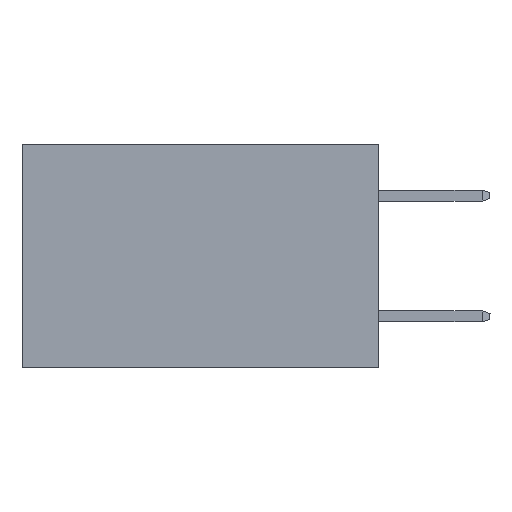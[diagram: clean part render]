
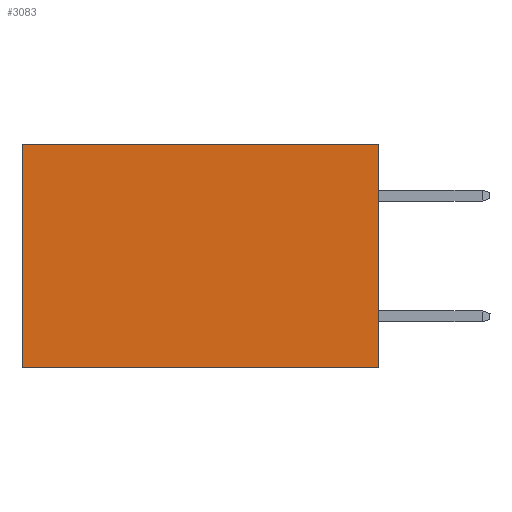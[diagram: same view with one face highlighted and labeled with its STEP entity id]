
A CAD part, left-side view. The second image highlights one B-rep face of the part: STEP entity #3083.
In plain terms, the highlighted planar face has unit normal (-1, 0, 0).
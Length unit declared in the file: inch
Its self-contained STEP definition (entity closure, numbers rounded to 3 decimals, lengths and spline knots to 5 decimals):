
#747 = DIRECTION ( 'NONE',  ( 0., 0., -1. ) ) ;
#791 = LINE ( 'NONE', #6484, #8474 ) ;
#910 = CARTESIAN_POINT ( 'NONE',  ( 0.277, 0.59, -0.37 ) ) ;
#1639 = CARTESIAN_POINT ( 'NONE',  ( 0.277, 0., -0.37 ) ) ;
#1869 = EDGE_CURVE ( 'NONE', #4061, #5436, #791, .T. ) ;
#1875 = VECTOR ( 'NONE', #5075, 39.37008 ) ;
#2324 = LINE ( 'NONE', #5632, #4254 ) ;
#2449 = EDGE_LOOP ( 'NONE', ( #4635, #6567, #8418, #2709 ) ) ;
#2709 = ORIENTED_EDGE ( 'NONE', *, *, #1869, .T. ) ;
#2907 = VECTOR ( 'NONE', #747, 39.37008 ) ;
#3083 = ADVANCED_FACE ( 'NONE', ( #7697 ), #7698, .F. ) ;
#3632 = AXIS2_PLACEMENT_3D ( 'NONE', #7762, #5878, #5810 ) ;
#3664 = EDGE_CURVE ( 'NONE', #4647, #9461, #2324, .T. ) ;
#3695 = EDGE_CURVE ( 'NONE', #4061, #4647, #6456, .T. ) ;
#4061 = VERTEX_POINT ( 'NONE', #4425 ) ;
#4254 = VECTOR ( 'NONE', #5204, 39.37008 ) ;
#4349 = CARTESIAN_POINT ( 'NONE',  ( 0.277, 0.59, 0. ) ) ;
#4425 = CARTESIAN_POINT ( 'NONE',  ( 0.277, 0., 0. ) ) ;
#4635 = ORIENTED_EDGE ( 'NONE', *, *, #5919, .T. ) ;
#4647 = VERTEX_POINT ( 'NONE', #1639 ) ;
#5007 = CARTESIAN_POINT ( 'NONE',  ( 0.277, 0., -0.37 ) ) ;
#5075 = DIRECTION ( 'NONE',  ( 0., 0., -1. ) ) ;
#5204 = DIRECTION ( 'NONE',  ( 0., 1., 0. ) ) ;
#5436 = VERTEX_POINT ( 'NONE', #4349 ) ;
#5632 = CARTESIAN_POINT ( 'NONE',  ( 0.277, 0., -0.37 ) ) ;
#5810 = DIRECTION ( 'NONE',  ( 0., 0., -1. ) ) ;
#5878 = DIRECTION ( 'NONE',  ( 1., 0., 0. ) ) ;
#5919 = EDGE_CURVE ( 'NONE', #5436, #9461, #6988, .T. ) ;
#6456 = LINE ( 'NONE', #5007, #1875 ) ;
#6484 = CARTESIAN_POINT ( 'NONE',  ( 0.277, 0., 0. ) ) ;
#6567 = ORIENTED_EDGE ( 'NONE', *, *, #3664, .F. ) ;
#6894 = DIRECTION ( 'NONE',  ( 0., 1., 0. ) ) ;
#6988 = LINE ( 'NONE', #910, #2907 ) ;
#7697 = FACE_OUTER_BOUND ( 'NONE', #2449, .T. ) ;
#7698 = PLANE ( 'NONE',  #3632 ) ;
#7762 = CARTESIAN_POINT ( 'NONE',  ( 0.277, 0., -0.37 ) ) ;
#8418 = ORIENTED_EDGE ( 'NONE', *, *, #3695, .F. ) ;
#8474 = VECTOR ( 'NONE', #6894, 39.37008 ) ;
#9429 = CARTESIAN_POINT ( 'NONE',  ( 0.277, 0.59, -0.37 ) ) ;
#9461 = VERTEX_POINT ( 'NONE', #9429 ) ;
